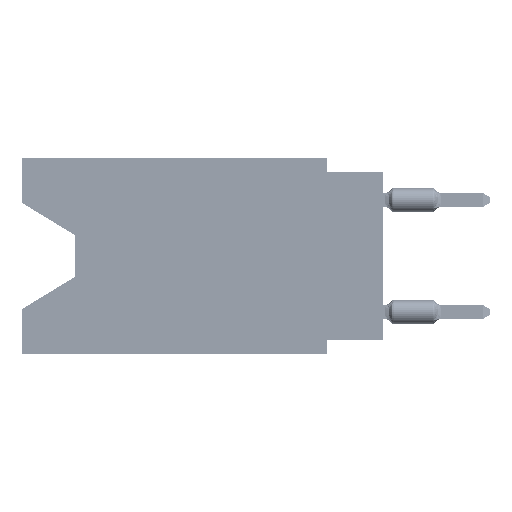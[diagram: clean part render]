
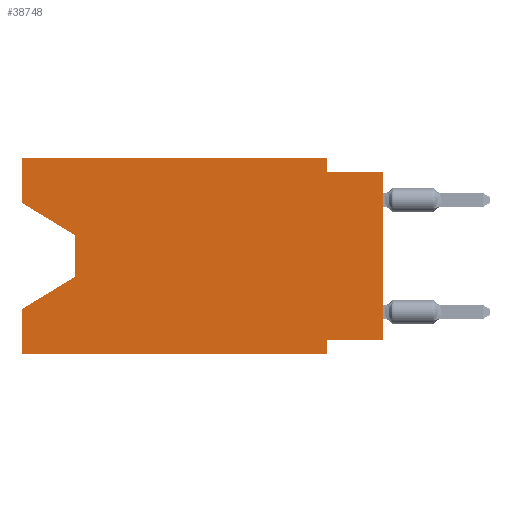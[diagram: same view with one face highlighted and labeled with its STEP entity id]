
A CAD part, left-side view. The second image highlights one B-rep face of the part: STEP entity #38748.
In plain terms, the highlighted planar face has unit normal (-1, 0, 0).
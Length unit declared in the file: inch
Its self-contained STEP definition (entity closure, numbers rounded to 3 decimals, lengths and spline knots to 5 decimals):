
#237 = LINE ( 'NONE', #42971, #10046 ) ;
#1363 = EDGE_CURVE ( 'NONE', #54865, #60712, #237, .T. ) ;
#1607 = EDGE_CURVE ( 'NONE', #45607, #58448, #35900, .T. ) ;
#2323 = VERTEX_POINT ( 'NONE', #6376 ) ;
#2652 = EDGE_CURVE ( 'NONE', #53970, #23734, #48017, .T. ) ;
#3091 = CARTESIAN_POINT ( 'NONE',  ( 0., 0.645, 0. ) ) ;
#3347 = CARTESIAN_POINT ( 'NONE',  ( 0., 0.1, 0. ) ) ;
#3399 = DIRECTION ( 'NONE',  ( 0., 0.855, -0.519 ) ) ;
#3624 = LINE ( 'NONE', #47060, #46325 ) ;
#4337 = CARTESIAN_POINT ( 'NONE',  ( 0., 0., -0.025 ) ) ;
#4687 = DIRECTION ( 'NONE',  ( 0., -1., 0. ) ) ;
#5351 = AXIS2_PLACEMENT_3D ( 'NONE', #3091, #61961, #67573 ) ;
#6376 = CARTESIAN_POINT ( 'NONE',  ( 0., 0.645, -0.26975 ) ) ;
#8792 = CARTESIAN_POINT ( 'NONE',  ( 0., 0.1, -0.35 ) ) ;
#9264 = CARTESIAN_POINT ( 'NONE',  ( 0., 0.1, -0.35 ) ) ;
#9475 = CARTESIAN_POINT ( 'NONE',  ( 0., 0.55, -0.138 ) ) ;
#9733 = CARTESIAN_POINT ( 'NONE',  ( 0., 0.645, -0.35 ) ) ;
#10046 = VECTOR ( 'NONE', #43657, 39.37008 ) ;
#10321 = ORIENTED_EDGE ( 'NONE', *, *, #25308, .F. ) ;
#11177 = CARTESIAN_POINT ( 'NONE',  ( 0., 0.1, -0.325 ) ) ;
#11695 = LINE ( 'NONE', #21523, #25045 ) ;
#12022 = VECTOR ( 'NONE', #4687, 39.37008 ) ;
#15300 = LINE ( 'NONE', #57717, #56140 ) ;
#16180 = EDGE_CURVE ( 'NONE', #58218, #38606, #35995, .T. ) ;
#17350 = VERTEX_POINT ( 'NONE', #3347 ) ;
#19297 = ORIENTED_EDGE ( 'NONE', *, *, #1607, .T. ) ;
#19544 = DIRECTION ( 'NONE',  ( 0., 1., 0. ) ) ;
#20818 = EDGE_CURVE ( 'NONE', #60712, #17350, #51249, .T. ) ;
#21523 = CARTESIAN_POINT ( 'NONE',  ( 0., 0.1, 0. ) ) ;
#21721 = EDGE_CURVE ( 'NONE', #54865, #53970, #15300, .T. ) ;
#22308 = ORIENTED_EDGE ( 'NONE', *, *, #30136, .T. ) ;
#22435 = EDGE_CURVE ( 'NONE', #38606, #58448, #47107, .T. ) ;
#22989 = ORIENTED_EDGE ( 'NONE', *, *, #22435, .F. ) ;
#23734 = VERTEX_POINT ( 'NONE', #63047 ) ;
#23886 = CARTESIAN_POINT ( 'NONE',  ( 0., 0.55, -0.138 ) ) ;
#24723 = VECTOR ( 'NONE', #36145, 39.37008 ) ;
#24803 = PLANE ( 'NONE',  #5351 ) ;
#25045 = VECTOR ( 'NONE', #59703, 39.37008 ) ;
#25123 = DIRECTION ( 'NONE',  ( 0., 0., 1. ) ) ;
#25308 = EDGE_CURVE ( 'NONE', #45607, #2323, #62282, .T. ) ;
#25375 = CARTESIAN_POINT ( 'NONE',  ( 0., 0.645, -0.35 ) ) ;
#27323 = ORIENTED_EDGE ( 'NONE', *, *, #57858, .F. ) ;
#30136 = EDGE_CURVE ( 'NONE', #23734, #2323, #61914, .T. ) ;
#30221 = ORIENTED_EDGE ( 'NONE', *, *, #44705, .T. ) ;
#30235 = VERTEX_POINT ( 'NONE', #52107 ) ;
#30690 = EDGE_LOOP ( 'NONE', ( #38607, #62944, #22308, #10321, #19297, #22989, #45017, #30221, #63814, #27323, #63182, #61886 ) ) ;
#33516 = VECTOR ( 'NONE', #19544, 39.37008 ) ;
#35004 = VECTOR ( 'NONE', #25123, 39.37008 ) ;
#35611 = CARTESIAN_POINT ( 'NONE',  ( 0., 0.55, -0.212 ) ) ;
#35662 = FACE_OUTER_BOUND ( 'NONE', #30690, .T. ) ;
#35900 = LINE ( 'NONE', #25375, #50738 ) ;
#35995 = LINE ( 'NONE', #58074, #33516 ) ;
#36145 = DIRECTION ( 'NONE',  ( 0., -1., 0. ) ) ;
#36580 = DIRECTION ( 'NONE',  ( 0., 0., -1. ) ) ;
#37963 = EDGE_CURVE ( 'NONE', #30235, #47118, #63201, .T. ) ;
#38606 = VERTEX_POINT ( 'NONE', #11177 ) ;
#38607 = ORIENTED_EDGE ( 'NONE', *, *, #21721, .T. ) ;
#38748 = ADVANCED_FACE ( 'NONE', ( #35662 ), #24803, .F. ) ;
#41603 = CARTESIAN_POINT ( 'NONE',  ( 0., 0.645, 0. ) ) ;
#42971 = CARTESIAN_POINT ( 'NONE',  ( 0., 0.645, 0. ) ) ;
#42986 = DIRECTION ( 'NONE',  ( 0., -0.855, -0.519 ) ) ;
#43657 = DIRECTION ( 'NONE',  ( 0., 0., 1. ) ) ;
#43699 = CARTESIAN_POINT ( 'NONE',  ( 0., 0.645, 0. ) ) ;
#44705 = EDGE_CURVE ( 'NONE', #58218, #47118, #3624, .T. ) ;
#45017 = ORIENTED_EDGE ( 'NONE', *, *, #16180, .F. ) ;
#45607 = VERTEX_POINT ( 'NONE', #9733 ) ;
#46325 = VECTOR ( 'NONE', #52315, 39.37008 ) ;
#47056 = CARTESIAN_POINT ( 'NONE',  ( 0., 0., -0.325 ) ) ;
#47060 = CARTESIAN_POINT ( 'NONE',  ( 0., 0., 0. ) ) ;
#47092 = VECTOR ( 'NONE', #36580, 39.37008 ) ;
#47107 = LINE ( 'NONE', #9264, #47092 ) ;
#47118 = VERTEX_POINT ( 'NONE', #53586 ) ;
#48017 = LINE ( 'NONE', #9475, #59777 ) ;
#50738 = VECTOR ( 'NONE', #68478, 39.37008 ) ;
#51249 = LINE ( 'NONE', #68382, #24723 ) ;
#52107 = CARTESIAN_POINT ( 'NONE',  ( 0., 0.1, -0.025 ) ) ;
#52315 = DIRECTION ( 'NONE',  ( 0., 0., 1. ) ) ;
#53586 = CARTESIAN_POINT ( 'NONE',  ( 0., 0., -0.025 ) ) ;
#53970 = VERTEX_POINT ( 'NONE', #23886 ) ;
#54865 = VERTEX_POINT ( 'NONE', #67413 ) ;
#56140 = VECTOR ( 'NONE', #42986, 39.37008 ) ;
#57717 = CARTESIAN_POINT ( 'NONE',  ( 0., 0.645, -0.08025 ) ) ;
#57858 = EDGE_CURVE ( 'NONE', #17350, #30235, #11695, .T. ) ;
#58074 = CARTESIAN_POINT ( 'NONE',  ( 0., 0., -0.325 ) ) ;
#58218 = VERTEX_POINT ( 'NONE', #47056 ) ;
#58448 = VERTEX_POINT ( 'NONE', #8792 ) ;
#59703 = DIRECTION ( 'NONE',  ( 0., 0., -1. ) ) ;
#59777 = VECTOR ( 'NONE', #68695, 39.37008 ) ;
#60712 = VERTEX_POINT ( 'NONE', #43699 ) ;
#61024 = VECTOR ( 'NONE', #3399, 39.37008 ) ;
#61886 = ORIENTED_EDGE ( 'NONE', *, *, #1363, .F. ) ;
#61914 = LINE ( 'NONE', #35611, #61024 ) ;
#61961 = DIRECTION ( 'NONE',  ( 1., 0., 0. ) ) ;
#62282 = LINE ( 'NONE', #41603, #35004 ) ;
#62944 = ORIENTED_EDGE ( 'NONE', *, *, #2652, .T. ) ;
#63047 = CARTESIAN_POINT ( 'NONE',  ( 0., 0.55, -0.212 ) ) ;
#63182 = ORIENTED_EDGE ( 'NONE', *, *, #20818, .F. ) ;
#63201 = LINE ( 'NONE', #4337, #12022 ) ;
#63814 = ORIENTED_EDGE ( 'NONE', *, *, #37963, .F. ) ;
#67413 = CARTESIAN_POINT ( 'NONE',  ( 0., 0.645, -0.08025 ) ) ;
#67573 = DIRECTION ( 'NONE',  ( 0., 0., -1. ) ) ;
#68382 = CARTESIAN_POINT ( 'NONE',  ( 0., 0.645, 0. ) ) ;
#68478 = DIRECTION ( 'NONE',  ( 0., -1., 0. ) ) ;
#68695 = DIRECTION ( 'NONE',  ( 0., 0., -1. ) ) ;
